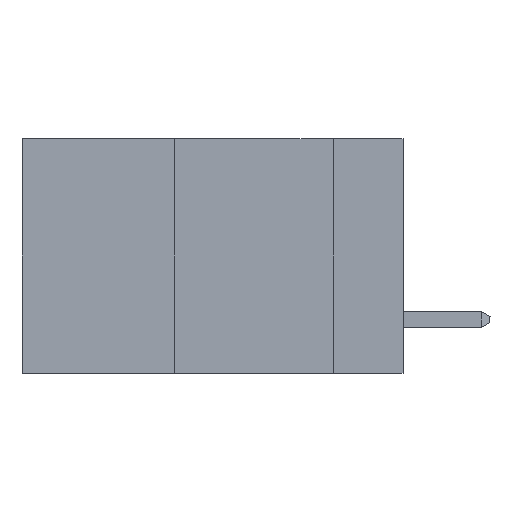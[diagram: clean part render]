
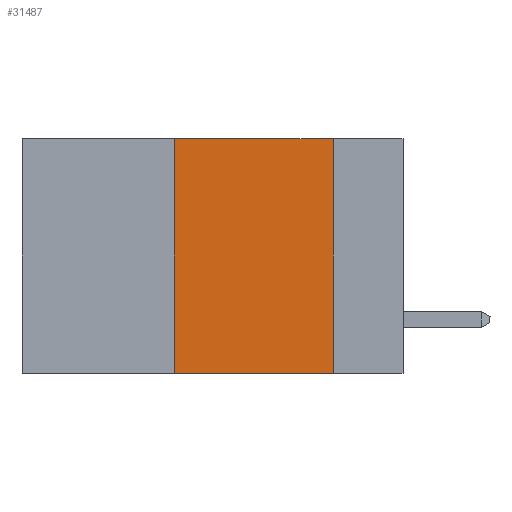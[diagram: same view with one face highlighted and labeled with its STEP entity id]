
A CAD part, left-side view. The second image highlights one B-rep face of the part: STEP entity #31487.
In plain terms, the highlighted planar face has unit normal (-1, 0, 0).
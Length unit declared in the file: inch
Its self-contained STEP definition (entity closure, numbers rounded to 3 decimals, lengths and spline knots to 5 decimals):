
#37 = PLANE ( 'NONE',  #25351 ) ;
#627 = VERTEX_POINT ( 'NONE', #10800 ) ;
#1329 = CARTESIAN_POINT ( 'NONE',  ( 0., 0.11, 0. ) ) ;
#2493 = EDGE_CURVE ( 'NONE', #18871, #15965, #37139, .T. ) ;
#2818 = FACE_OUTER_BOUND ( 'NONE', #20814, .T. ) ;
#5550 = CARTESIAN_POINT ( 'NONE',  ( 0., 0.11, 0. ) ) ;
#6232 = DIRECTION ( 'NONE',  ( 1., 0., 0. ) ) ;
#7962 = CARTESIAN_POINT ( 'NONE',  ( 0., 0.36, 0. ) ) ;
#8766 = DIRECTION ( 'NONE',  ( 0., 0., -1. ) ) ;
#10049 = CARTESIAN_POINT ( 'NONE',  ( 0., 0.6, 0. ) ) ;
#10092 = CARTESIAN_POINT ( 'NONE',  ( 0., 0.6, 0. ) ) ;
#10754 = EDGE_CURVE ( 'NONE', #627, #39795, #37483, .T. ) ;
#10800 = CARTESIAN_POINT ( 'NONE',  ( 0., 0.36, 0. ) ) ;
#10974 = CARTESIAN_POINT ( 'NONE',  ( 0., 0.36, -0.37 ) ) ;
#11453 = VECTOR ( 'NONE', #17310, 39.37008 ) ;
#14172 = EDGE_CURVE ( 'NONE', #39795, #15965, #26864, .T. ) ;
#14324 = ORIENTED_EDGE ( 'NONE', *, *, #10754, .F. ) ;
#15391 = VECTOR ( 'NONE', #37347, 39.37008 ) ;
#15965 = VERTEX_POINT ( 'NONE', #24681 ) ;
#17310 = DIRECTION ( 'NONE',  ( 0., 0., 1. ) ) ;
#18174 = CARTESIAN_POINT ( 'NONE',  ( 0., 0.6, -0.37 ) ) ;
#18190 = ORIENTED_EDGE ( 'NONE', *, *, #37877, .F. ) ;
#18871 = VERTEX_POINT ( 'NONE', #10974 ) ;
#19400 = DIRECTION ( 'NONE',  ( 0., 0., -1. ) ) ;
#20814 = EDGE_LOOP ( 'NONE', ( #32433, #14324, #18190, #29122 ) ) ;
#23038 = DIRECTION ( 'NONE',  ( 0., -1., 0. ) ) ;
#24526 = VECTOR ( 'NONE', #23038, 39.37008 ) ;
#24681 = CARTESIAN_POINT ( 'NONE',  ( 0., 0.11, -0.37 ) ) ;
#25351 = AXIS2_PLACEMENT_3D ( 'NONE', #10049, #6232, #19400 ) ;
#26864 = LINE ( 'NONE', #1329, #39325 ) ;
#29122 = ORIENTED_EDGE ( 'NONE', *, *, #2493, .T. ) ;
#31487 = ADVANCED_FACE ( 'NONE', ( #2818 ), #37, .F. ) ;
#32433 = ORIENTED_EDGE ( 'NONE', *, *, #14172, .F. ) ;
#37139 = LINE ( 'NONE', #18174, #15391 ) ;
#37347 = DIRECTION ( 'NONE',  ( 0., -1., 0. ) ) ;
#37483 = LINE ( 'NONE', #10092, #24526 ) ;
#37877 = EDGE_CURVE ( 'NONE', #18871, #627, #39671, .T. ) ;
#39325 = VECTOR ( 'NONE', #8766, 39.37008 ) ;
#39671 = LINE ( 'NONE', #7962, #11453 ) ;
#39795 = VERTEX_POINT ( 'NONE', #5550 ) ;
